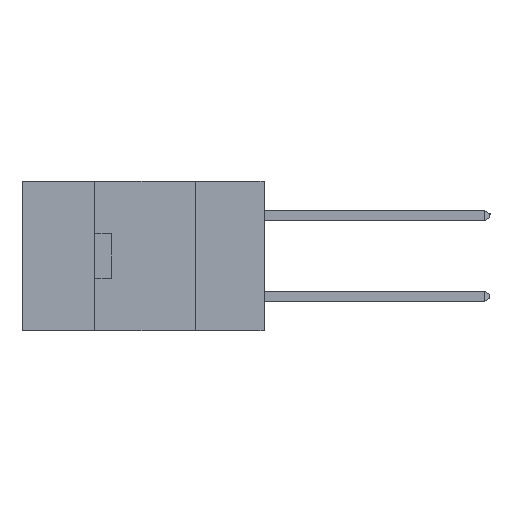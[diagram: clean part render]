
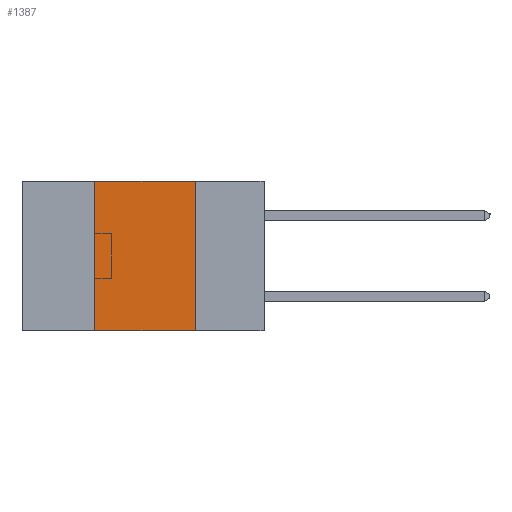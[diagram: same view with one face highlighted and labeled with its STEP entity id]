
A CAD part, left-side view. The second image highlights one B-rep face of the part: STEP entity #1387.
In plain terms, the highlighted planar face has unit normal (-1, 0, 0).
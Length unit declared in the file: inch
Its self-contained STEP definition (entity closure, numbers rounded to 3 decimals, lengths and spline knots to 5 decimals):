
#74 = DIRECTION ( 'NONE',  ( 0., -1., 0. ) ) ;
#94 = DIRECTION ( 'NONE',  ( 0., 0., -1. ) ) ;
#729 = ORIENTED_EDGE ( 'NONE', *, *, #16322, .T. ) ;
#1283 = VECTOR ( 'NONE', #94, 39.37008 ) ;
#1387 = ADVANCED_FACE ( 'NONE', ( #20184 ), #26912, .F. ) ;
#1654 = EDGE_CURVE ( 'NONE', #24032, #18603, #10624, .T. ) ;
#1708 = LINE ( 'NONE', #19856, #1283 ) ;
#4133 = EDGE_LOOP ( 'NONE', ( #7377, #20629, #24579, #729 ) ) ;
#4342 = CARTESIAN_POINT ( 'NONE',  ( 0., 0.6, 0. ) ) ;
#4388 = CARTESIAN_POINT ( 'NONE',  ( 0., 0.42, 0. ) ) ;
#5236 = VECTOR ( 'NONE', #12524, 39.37008 ) ;
#7269 = VECTOR ( 'NONE', #74, 39.37008 ) ;
#7377 = ORIENTED_EDGE ( 'NONE', *, *, #24663, .F. ) ;
#7798 = CARTESIAN_POINT ( 'NONE',  ( 0., 0.6, 0. ) ) ;
#9262 = LINE ( 'NONE', #9568, #7269 ) ;
#9469 = CARTESIAN_POINT ( 'NONE',  ( 0., 0.17, -0.37 ) ) ;
#9568 = CARTESIAN_POINT ( 'NONE',  ( 0., 0.6, -0.37 ) ) ;
#9887 = EDGE_CURVE ( 'NONE', #18603, #22916, #16278, .T. ) ;
#10624 = LINE ( 'NONE', #14728, #5236 ) ;
#12524 = DIRECTION ( 'NONE',  ( 0., 0., 1. ) ) ;
#12701 = VECTOR ( 'NONE', #25668, 39.37008 ) ;
#14728 = CARTESIAN_POINT ( 'NONE',  ( 0., 0.42, -0.37 ) ) ;
#16278 = LINE ( 'NONE', #7798, #12701 ) ;
#16322 = EDGE_CURVE ( 'NONE', #24032, #19185, #9262, .T. ) ;
#17820 = DIRECTION ( 'NONE',  ( 0., 0., -1. ) ) ;
#18603 = VERTEX_POINT ( 'NONE', #4388 ) ;
#19106 = CARTESIAN_POINT ( 'NONE',  ( 0., 0.17, 0. ) ) ;
#19185 = VERTEX_POINT ( 'NONE', #9469 ) ;
#19856 = CARTESIAN_POINT ( 'NONE',  ( 0., 0.17, -0.37 ) ) ;
#20184 = FACE_OUTER_BOUND ( 'NONE', #4133, .T. ) ;
#20326 = DIRECTION ( 'NONE',  ( 1., 0., 0. ) ) ;
#20629 = ORIENTED_EDGE ( 'NONE', *, *, #9887, .F. ) ;
#22916 = VERTEX_POINT ( 'NONE', #19106 ) ;
#23582 = AXIS2_PLACEMENT_3D ( 'NONE', #4342, #20326, #17820 ) ;
#24032 = VERTEX_POINT ( 'NONE', #25911 ) ;
#24579 = ORIENTED_EDGE ( 'NONE', *, *, #1654, .F. ) ;
#24663 = EDGE_CURVE ( 'NONE', #22916, #19185, #1708, .T. ) ;
#25668 = DIRECTION ( 'NONE',  ( 0., -1., 0. ) ) ;
#25911 = CARTESIAN_POINT ( 'NONE',  ( 0., 0.42, -0.37 ) ) ;
#26912 = PLANE ( 'NONE',  #23582 ) ;
